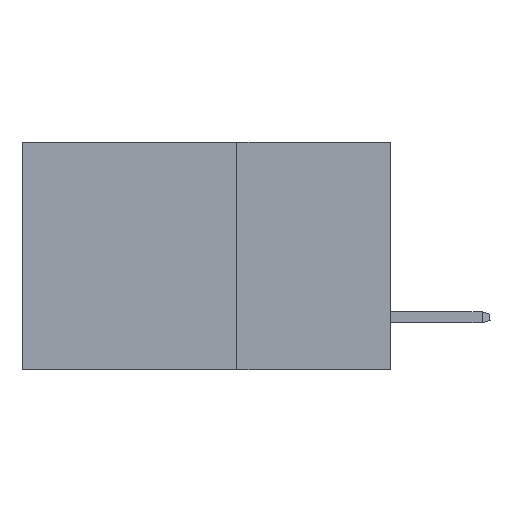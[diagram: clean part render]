
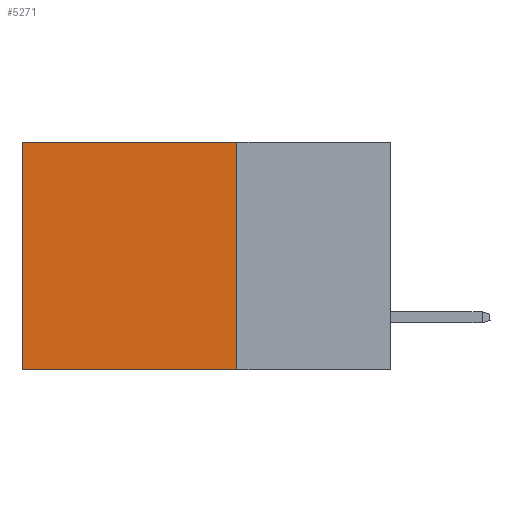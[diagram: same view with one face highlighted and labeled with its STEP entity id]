
A CAD part, left-side view. The second image highlights one B-rep face of the part: STEP entity #5271.
In plain terms, the highlighted planar face has unit normal (-1, 0, 0).
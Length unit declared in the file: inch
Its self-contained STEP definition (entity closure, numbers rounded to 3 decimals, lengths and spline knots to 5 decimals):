
#408 = CARTESIAN_POINT ( 'NONE',  ( 0.2875, 0.25, -0.37 ) ) ;
#719 = CARTESIAN_POINT ( 'NONE',  ( 0.2875, 0.25, -0.37 ) ) ;
#766 = DIRECTION ( 'NONE',  ( 0., 1., 0. ) ) ;
#822 = CARTESIAN_POINT ( 'NONE',  ( 0.2875, 0.25, 0. ) ) ;
#1117 = EDGE_LOOP ( 'NONE', ( #15594, #9174, #5168, #13454 ) ) ;
#1618 = VERTEX_POINT ( 'NONE', #719 ) ;
#1913 = EDGE_CURVE ( 'NONE', #18240, #17943, #3291, .T. ) ;
#2034 = DIRECTION ( 'NONE',  ( 0., 1., 0. ) ) ;
#2280 = CARTESIAN_POINT ( 'NONE',  ( 0.2875, 0.25, 0. ) ) ;
#3291 = LINE ( 'NONE', #822, #6660 ) ;
#3397 = DIRECTION ( 'NONE',  ( 1., 0., 0. ) ) ;
#3840 = EDGE_CURVE ( 'NONE', #17943, #7171, #17204, .T. ) ;
#4792 = PLANE ( 'NONE',  #9160 ) ;
#4847 = CARTESIAN_POINT ( 'NONE',  ( 0.2875, 0.6, 0. ) ) ;
#4856 = DIRECTION ( 'NONE',  ( 0., 0., -1. ) ) ;
#5120 = EDGE_CURVE ( 'NONE', #18240, #1618, #8532, .T. ) ;
#5168 = ORIENTED_EDGE ( 'NONE', *, *, #5120, .F. ) ;
#5271 = ADVANCED_FACE ( 'NONE', ( #12574 ), #4792, .F. ) ;
#6294 = VECTOR ( 'NONE', #11001, 39.37008 ) ;
#6348 = VECTOR ( 'NONE', #13591, 39.37008 ) ;
#6660 = VECTOR ( 'NONE', #766, 39.37008 ) ;
#7171 = VERTEX_POINT ( 'NONE', #7570 ) ;
#7570 = CARTESIAN_POINT ( 'NONE',  ( 0.2875, 0.6, -0.37 ) ) ;
#8532 = LINE ( 'NONE', #10880, #6294 ) ;
#9160 = AXIS2_PLACEMENT_3D ( 'NONE', #10611, #3397, #4856 ) ;
#9174 = ORIENTED_EDGE ( 'NONE', *, *, #14413, .F. ) ;
#10611 = CARTESIAN_POINT ( 'NONE',  ( 0.2875, 0.25, 0. ) ) ;
#10880 = CARTESIAN_POINT ( 'NONE',  ( 0.2875, 0.25, 0. ) ) ;
#11001 = DIRECTION ( 'NONE',  ( 0., 0., -1. ) ) ;
#12574 = FACE_OUTER_BOUND ( 'NONE', #1117, .T. ) ;
#13454 = ORIENTED_EDGE ( 'NONE', *, *, #1913, .T. ) ;
#13591 = DIRECTION ( 'NONE',  ( 0., 0., -1. ) ) ;
#14386 = LINE ( 'NONE', #408, #16652 ) ;
#14413 = EDGE_CURVE ( 'NONE', #1618, #7171, #14386, .T. ) ;
#15288 = CARTESIAN_POINT ( 'NONE',  ( 0.2875, 0.6, 0. ) ) ;
#15594 = ORIENTED_EDGE ( 'NONE', *, *, #3840, .T. ) ;
#16652 = VECTOR ( 'NONE', #2034, 39.37008 ) ;
#17204 = LINE ( 'NONE', #4847, #6348 ) ;
#17943 = VERTEX_POINT ( 'NONE', #15288 ) ;
#18240 = VERTEX_POINT ( 'NONE', #2280 ) ;
